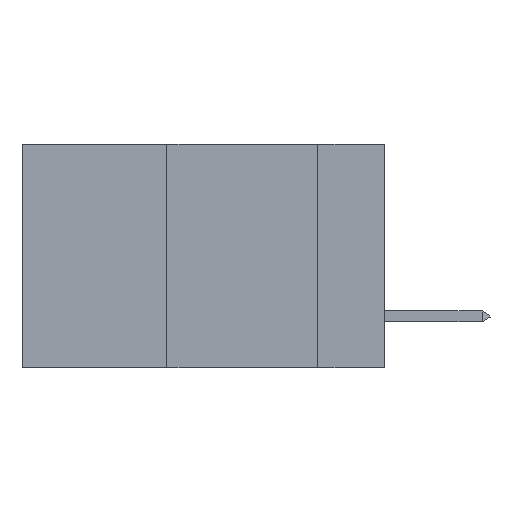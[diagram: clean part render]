
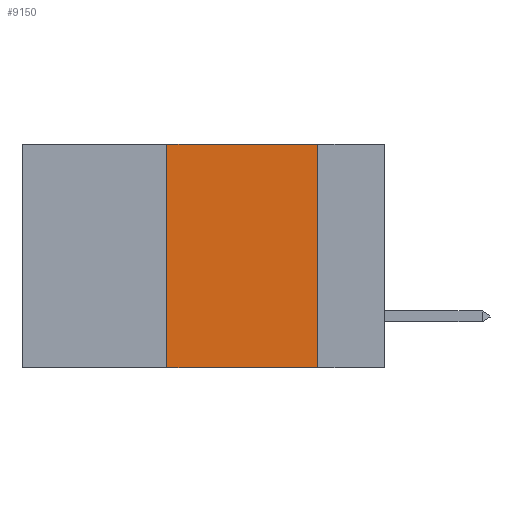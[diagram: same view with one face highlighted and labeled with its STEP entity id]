
A CAD part, left-side view. The second image highlights one B-rep face of the part: STEP entity #9150.
In plain terms, the highlighted planar face has unit normal (-1, 0, 0).
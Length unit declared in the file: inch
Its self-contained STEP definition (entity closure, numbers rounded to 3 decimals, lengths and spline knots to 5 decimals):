
#494 = DIRECTION ( 'NONE',  ( 0., 0., 1. ) ) ;
#1009 = CARTESIAN_POINT ( 'NONE',  ( 0., 0.11, 0. ) ) ;
#1428 = FACE_OUTER_BOUND ( 'NONE', #10243, .T. ) ;
#1955 = VECTOR ( 'NONE', #494, 39.37008 ) ;
#2304 = LINE ( 'NONE', #5054, #1955 ) ;
#2656 = LINE ( 'NONE', #10319, #6876 ) ;
#2973 = EDGE_CURVE ( 'NONE', #11577, #13874, #2656, .T. ) ;
#3178 = DIRECTION ( 'NONE',  ( 0., 0., -1. ) ) ;
#3350 = DIRECTION ( 'NONE',  ( 0., -1., 0. ) ) ;
#3967 = VECTOR ( 'NONE', #12727, 39.37008 ) ;
#4097 = EDGE_CURVE ( 'NONE', #11604, #13874, #6847, .T. ) ;
#4156 = AXIS2_PLACEMENT_3D ( 'NONE', #10652, #4203, #3178 ) ;
#4203 = DIRECTION ( 'NONE',  ( 1., 0., 0. ) ) ;
#4563 = EDGE_CURVE ( 'NONE', #11577, #6004, #2304, .T. ) ;
#5054 = CARTESIAN_POINT ( 'NONE',  ( 0., 0.36, 0. ) ) ;
#5343 = CARTESIAN_POINT ( 'NONE',  ( 0., 0.11, 0. ) ) ;
#6004 = VERTEX_POINT ( 'NONE', #6676 ) ;
#6370 = ORIENTED_EDGE ( 'NONE', *, *, #4097, .F. ) ;
#6676 = CARTESIAN_POINT ( 'NONE',  ( 0., 0.36, 0. ) ) ;
#6847 = LINE ( 'NONE', #5343, #3967 ) ;
#6876 = VECTOR ( 'NONE', #3350, 39.37008 ) ;
#7183 = CARTESIAN_POINT ( 'NONE',  ( 0., 0.36, -0.37 ) ) ;
#7359 = LINE ( 'NONE', #13465, #13859 ) ;
#7824 = ORIENTED_EDGE ( 'NONE', *, *, #4563, .F. ) ;
#7975 = DIRECTION ( 'NONE',  ( 0., -1., 0. ) ) ;
#7984 = EDGE_CURVE ( 'NONE', #6004, #11604, #7359, .T. ) ;
#9106 = ORIENTED_EDGE ( 'NONE', *, *, #2973, .T. ) ;
#9150 = ADVANCED_FACE ( 'NONE', ( #1428 ), #9593, .F. ) ;
#9593 = PLANE ( 'NONE',  #4156 ) ;
#10243 = EDGE_LOOP ( 'NONE', ( #6370, #11748, #7824, #9106 ) ) ;
#10319 = CARTESIAN_POINT ( 'NONE',  ( 0., 0.6, -0.37 ) ) ;
#10652 = CARTESIAN_POINT ( 'NONE',  ( 0., 0.6, 0. ) ) ;
#10930 = CARTESIAN_POINT ( 'NONE',  ( 0., 0.11, -0.37 ) ) ;
#11577 = VERTEX_POINT ( 'NONE', #7183 ) ;
#11604 = VERTEX_POINT ( 'NONE', #1009 ) ;
#11748 = ORIENTED_EDGE ( 'NONE', *, *, #7984, .F. ) ;
#12727 = DIRECTION ( 'NONE',  ( 0., 0., -1. ) ) ;
#13465 = CARTESIAN_POINT ( 'NONE',  ( 0., 0.6, 0. ) ) ;
#13859 = VECTOR ( 'NONE', #7975, 39.37008 ) ;
#13874 = VERTEX_POINT ( 'NONE', #10930 ) ;
